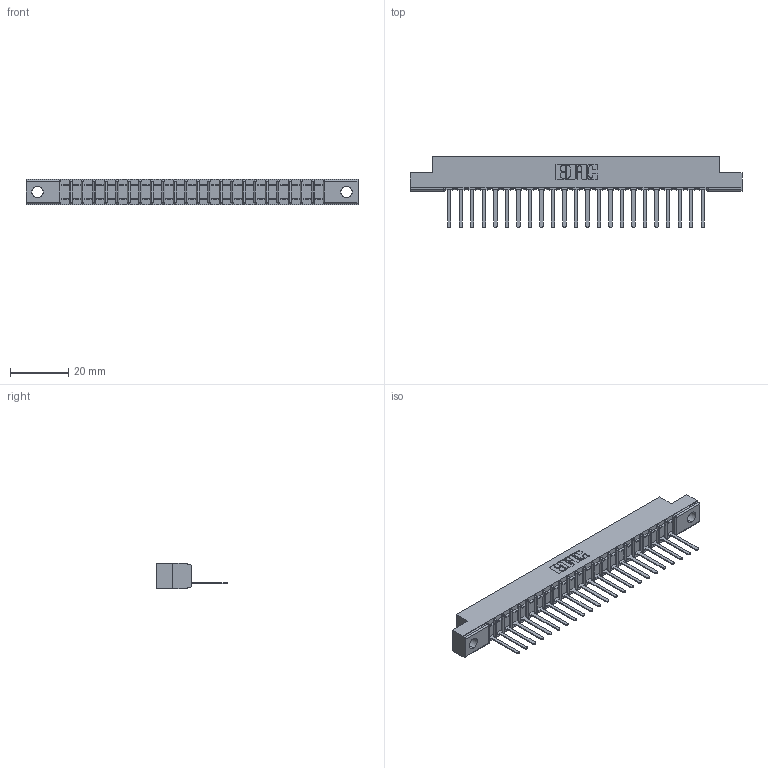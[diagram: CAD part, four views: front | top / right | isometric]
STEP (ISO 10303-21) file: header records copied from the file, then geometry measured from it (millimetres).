
FILE_DESCRIPTION (( 'STEP AP203' ), '1' );
FILE_NAME ('357-023-441-102.STEP', '2020-10-01T11:15:39', ( '' ), ( '' ), 'SwSTEP 2.0', 'SolidWorks 2020', '' );
FILE_SCHEMA (( 'CONFIG_CONTROL_DESIGN' ));
Length unit declared in the file: inch
Products named in the file (3): 307-290-002_541; 357-023-441-102; 307 Part_.128 Dia Mounting Holes
Assembly tree (24 placements, depth 2):
  357-023-441-102
    307 Part_.128 Dia Mounting Holes
    307-290-002_541  x23
Bounding box: 114.15 x 24.59 x 8.71 mm (x, y, z)
Volume: 7513.4 mm3; surface area: 13961.3 mm2
Topology: 24 solids, 24 shells, 1844 faces, 5659 edges, 3706 vertices
Faces by surface type: plane 1105, cylinder 691, sphere 48
Entity records: 22780 total; most frequent: CARTESIAN_POINT 3840, ORIENTED_EDGE 3830, DIRECTION 3739, EDGE_CURVE 1915, LINE 1457, VECTOR 1457, VERTEX_POINT 1242, AXIS2_PLACEMENT_3D 1141
